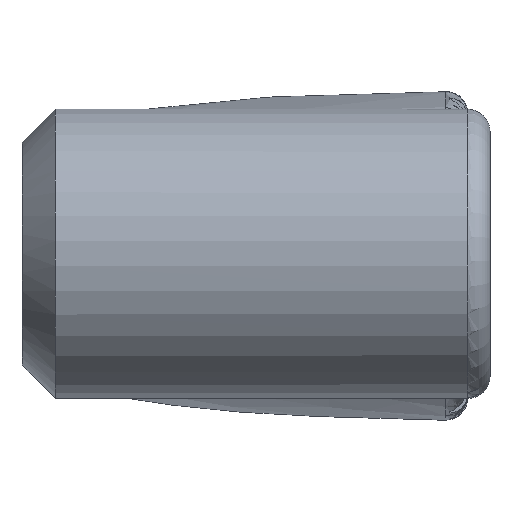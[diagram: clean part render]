
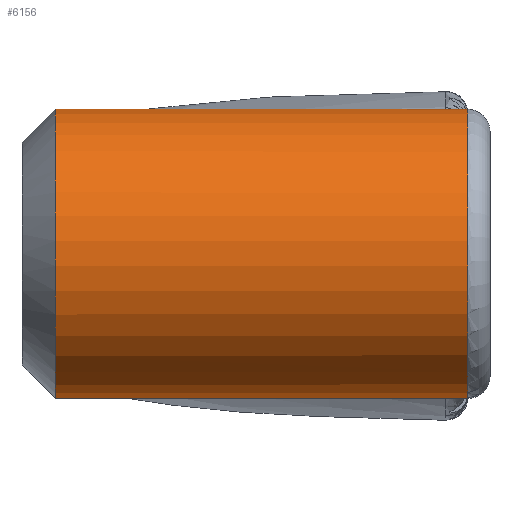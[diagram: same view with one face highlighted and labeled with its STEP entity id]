
A CAD part, top view. The second image highlights one B-rep face of the part: STEP entity #6156.
In plain terms, the highlighted cylindrical face has radius 6.5 mm (diameter 13 mm), a partial arc.
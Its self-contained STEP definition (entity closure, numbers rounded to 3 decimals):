
#26 = VERTEX_POINT ( 'NONE', #1759 ) ;
#194 = CARTESIAN_POINT ( 'NONE',  ( 62.179, 45.029, -26.587 ) ) ;
#346 = CARTESIAN_POINT ( 'NONE',  ( 62.179, 47.829, -20.721 ) ) ;
#421 = DIRECTION ( 'NONE',  ( 0., 0., -1. ) ) ;
#468 = CARTESIAN_POINT ( 'NONE',  ( 80.653, 49.889, -26.887 ) ) ;
#689 = CARTESIAN_POINT ( 'NONE',  ( 80.484, 45.423, -26.76 ) ) ;
#801 = VECTOR ( 'NONE', #3769, 1000. ) ;
#809 = VECTOR ( 'NONE', #3462, 1000. ) ;
#999 = CARTESIAN_POINT ( 'NONE',  ( 80.679, 49.629, -26.966 ) ) ;
#1005 = EDGE_CURVE ( 'NONE', #2440, #4852, #2086, .T. ) ;
#1162 = CARTESIAN_POINT ( 'NONE',  ( 79.949, 45.058, -26.6 ) ) ;
#1188 = DIRECTION ( 'NONE',  ( 1., 0., 0. ) ) ;
#1205 = CARTESIAN_POINT ( 'NONE',  ( 80.194, 45.162, -26.648 ) ) ;
#1381 = CARTESIAN_POINT ( 'NONE',  ( 75.679, 45.029, -26.587 ) ) ;
#1384 = DIRECTION ( 'NONE',  ( -1., 0., 0. ) ) ;
#1432 = CYLINDRICAL_SURFACE ( 'NONE', #2211, 6.5 ) ;
#1437 = CARTESIAN_POINT ( 'NONE',  ( 80.484, 50.236, -26.76 ) ) ;
#1586 = AXIS2_PLACEMENT_3D ( 'NONE', #5080, #1188, #2123 ) ;
#1672 = CARTESIAN_POINT ( 'NONE',  ( 79.679, 45.029, -26.587 ) ) ;
#1715 = LINE ( 'NONE', #6371, #809 ) ;
#1759 = CARTESIAN_POINT ( 'NONE',  ( 80.679, 46.029, -26.966 ) ) ;
#1791 = DIRECTION ( 'NONE',  ( -1., 0., 0. ) ) ;
#1798 = EDGE_CURVE ( 'NONE', #2097, #26, #3905, .T. ) ;
#2086 = LINE ( 'NONE', #1381, #801 ) ;
#2097 = VERTEX_POINT ( 'NONE', #4824 ) ;
#2104 = B_SPLINE_CURVE_WITH_KNOTS ( 'NONE', 3,
 ( #4626, #5520, #5430, #5893, #4414, #1437, #3977, #468, #3471, #999 ),
 .UNSPECIFIED., .F., .F.,
 ( 4, 2, 2, 2, 4 ),
 ( 0., 0., 0.001, 0.001, 0.002 ),
 .UNSPECIFIED. ) ;
#2122 = CARTESIAN_POINT ( 'NONE',  ( 80.679, 46.029, -26.966 ) ) ;
#2123 = DIRECTION ( 'NONE',  ( 0., 0., -1. ) ) ;
#2165 = CIRCLE ( 'NONE', #4229, 6.5 ) ;
#2211 = AXIS2_PLACEMENT_3D ( 'NONE', #4793, #1791, #5286 ) ;
#2440 = VERTEX_POINT ( 'NONE', #1672 ) ;
#2596 = CARTESIAN_POINT ( 'NONE',  ( 79.815, 45.029, -26.587 ) ) ;
#3089 = EDGE_CURVE ( 'NONE', #5228, #4134, #1715, .T. ) ;
#3102 = CARTESIAN_POINT ( 'NONE',  ( 80.556, 45.533, -26.803 ) ) ;
#3223 = ORIENTED_EDGE ( 'NONE', *, *, #1005, .F. ) ;
#3335 = ORIENTED_EDGE ( 'NONE', *, *, #6030, .F. ) ;
#3337 = B_SPLINE_CURVE_WITH_KNOTS ( 'NONE', 3,
 ( #4168, #2596, #1162, #1205, #6033, #689, #3102, #4114, #4658, #2122 ),
 .UNSPECIFIED., .F., .F.,
 ( 4, 2, 2, 2, 4 ),
 ( 0., 0., 0.001, 0.001, 0.002 ),
 .UNSPECIFIED. ) ;
#3387 = EDGE_CURVE ( 'NONE', #2440, #26, #3337, .T. ) ;
#3462 = DIRECTION ( 'NONE',  ( 1., 0., 0. ) ) ;
#3471 = CARTESIAN_POINT ( 'NONE',  ( 80.679, 49.76, -26.929 ) ) ;
#3769 = DIRECTION ( 'NONE',  ( -1., 0., 0. ) ) ;
#3813 = ORIENTED_EDGE ( 'NONE', *, *, #4498, .F. ) ;
#3905 = CIRCLE ( 'NONE', #1586, 6.5 ) ;
#3977 = CARTESIAN_POINT ( 'NONE',  ( 80.556, 50.126, -26.803 ) ) ;
#4020 = CARTESIAN_POINT ( 'NONE',  ( 79.679, 50.629, -26.587 ) ) ;
#4114 = CARTESIAN_POINT ( 'NONE',  ( 80.653, 45.77, -26.887 ) ) ;
#4134 = VERTEX_POINT ( 'NONE', #4020 ) ;
#4168 = CARTESIAN_POINT ( 'NONE',  ( 79.679, 45.029, -26.587 ) ) ;
#4229 = AXIS2_PLACEMENT_3D ( 'NONE', #346, #1384, #421 ) ;
#4414 = CARTESIAN_POINT ( 'NONE',  ( 80.304, 50.421, -26.683 ) ) ;
#4485 = EDGE_LOOP ( 'NONE', ( #5314, #3335, #4721, #3813, #3223, #5901 ) ) ;
#4498 = EDGE_CURVE ( 'NONE', #4852, #5228, #2165, .T. ) ;
#4626 = CARTESIAN_POINT ( 'NONE',  ( 79.679, 50.629, -26.587 ) ) ;
#4658 = CARTESIAN_POINT ( 'NONE',  ( 80.679, 45.898, -26.929 ) ) ;
#4721 = ORIENTED_EDGE ( 'NONE', *, *, #3089, .F. ) ;
#4793 = CARTESIAN_POINT ( 'NONE',  ( 75.679, 47.829, -20.721 ) ) ;
#4824 = CARTESIAN_POINT ( 'NONE',  ( 80.679, 49.629, -26.966 ) ) ;
#4852 = VERTEX_POINT ( 'NONE', #194 ) ;
#5080 = CARTESIAN_POINT ( 'NONE',  ( 80.679, 47.829, -20.721 ) ) ;
#5228 = VERTEX_POINT ( 'NONE', #6330 ) ;
#5286 = DIRECTION ( 'NONE',  ( 0., 0., -1. ) ) ;
#5314 = ORIENTED_EDGE ( 'NONE', *, *, #1798, .F. ) ;
#5430 = CARTESIAN_POINT ( 'NONE',  ( 79.949, 50.601, -26.6 ) ) ;
#5520 = CARTESIAN_POINT ( 'NONE',  ( 79.815, 50.629, -26.587 ) ) ;
#5883 = FACE_OUTER_BOUND ( 'NONE', #4485, .T. ) ;
#5893 = CARTESIAN_POINT ( 'NONE',  ( 80.194, 50.497, -26.648 ) ) ;
#5901 = ORIENTED_EDGE ( 'NONE', *, *, #3387, .T. ) ;
#6030 = EDGE_CURVE ( 'NONE', #4134, #2097, #2104, .T. ) ;
#6033 = CARTESIAN_POINT ( 'NONE',  ( 80.304, 45.238, -26.683 ) ) ;
#6156 = ADVANCED_FACE ( 'NONE', ( #5883 ), #1432, .T. ) ;
#6330 = CARTESIAN_POINT ( 'NONE',  ( 62.179, 50.629, -26.587 ) ) ;
#6371 = CARTESIAN_POINT ( 'NONE',  ( 75.679, 50.629, -26.587 ) ) ;
